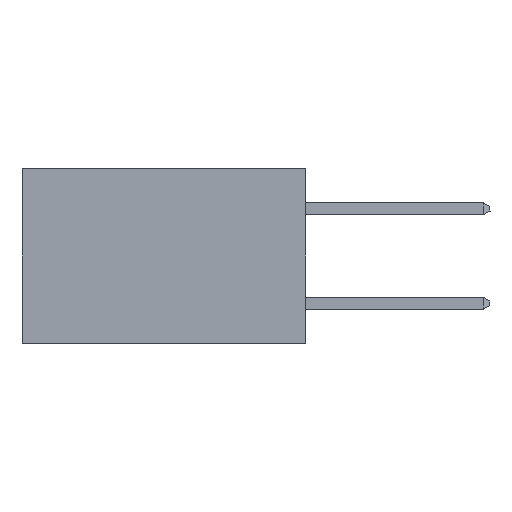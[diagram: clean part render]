
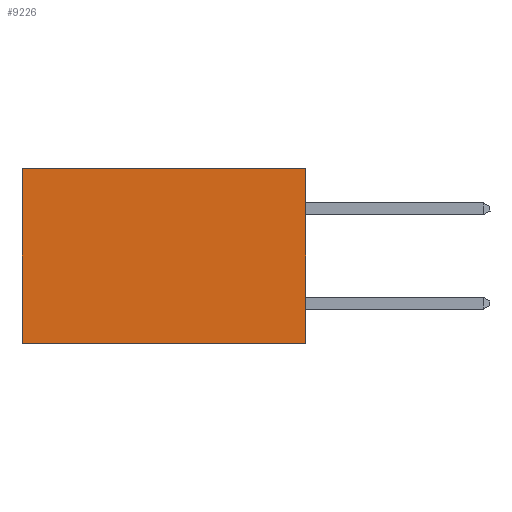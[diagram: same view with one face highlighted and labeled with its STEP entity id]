
A CAD part, left-side view. The second image highlights one B-rep face of the part: STEP entity #9226.
In plain terms, the highlighted planar face has unit normal (-1, 0, 0).
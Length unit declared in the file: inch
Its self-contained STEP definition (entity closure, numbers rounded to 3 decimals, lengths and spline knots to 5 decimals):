
#506 = DIRECTION ( 'NONE',  ( 0., 1., 0. ) ) ;
#550 = EDGE_CURVE ( 'NONE', #14783, #10719, #13028, .T. ) ;
#842 = EDGE_CURVE ( 'NONE', #10719, #13109, #15501, .T. ) ;
#994 = VECTOR ( 'NONE', #506, 39.37008 ) ;
#1002 = EDGE_CURVE ( 'NONE', #3822, #13109, #2439, .T. ) ;
#1236 = FACE_OUTER_BOUND ( 'NONE', #16399, .T. ) ;
#1296 = AXIS2_PLACEMENT_3D ( 'NONE', #7543, #8879, #3554 ) ;
#2439 = LINE ( 'NONE', #15503, #12427 ) ;
#3278 = ORIENTED_EDGE ( 'NONE', *, *, #842, .F. ) ;
#3554 = DIRECTION ( 'NONE',  ( 0., 0., -1. ) ) ;
#3822 = VERTEX_POINT ( 'NONE', #11795 ) ;
#5274 = CARTESIAN_POINT ( 'NONE',  ( 0.298, 0., 0. ) ) ;
#7299 = ORIENTED_EDGE ( 'NONE', *, *, #550, .F. ) ;
#7385 = ORIENTED_EDGE ( 'NONE', *, *, #14530, .T. ) ;
#7543 = CARTESIAN_POINT ( 'NONE',  ( 0.298, 0., 0. ) ) ;
#7677 = DIRECTION ( 'NONE',  ( 0., 0., -1. ) ) ;
#8879 = DIRECTION ( 'NONE',  ( 1., 0., 0. ) ) ;
#8981 = VECTOR ( 'NONE', #12242, 39.37008 ) ;
#9226 = ADVANCED_FACE ( 'NONE', ( #1236 ), #14047, .F. ) ;
#10137 = CARTESIAN_POINT ( 'NONE',  ( 0.298, 0., -0.37 ) ) ;
#10560 = CARTESIAN_POINT ( 'NONE',  ( 0.298, 0., 0. ) ) ;
#10681 = DIRECTION ( 'NONE',  ( 0., 0., -1. ) ) ;
#10719 = VERTEX_POINT ( 'NONE', #13956 ) ;
#10819 = VECTOR ( 'NONE', #10681, 39.37008 ) ;
#11795 = CARTESIAN_POINT ( 'NONE',  ( 0.298, 0.6, 0. ) ) ;
#11883 = CARTESIAN_POINT ( 'NONE',  ( 0.298, 0.6, -0.37 ) ) ;
#12242 = DIRECTION ( 'NONE',  ( 0., 1., 0. ) ) ;
#12427 = VECTOR ( 'NONE', #7677, 39.37008 ) ;
#13028 = LINE ( 'NONE', #10560, #10819 ) ;
#13109 = VERTEX_POINT ( 'NONE', #11883 ) ;
#13585 = LINE ( 'NONE', #15730, #994 ) ;
#13952 = ORIENTED_EDGE ( 'NONE', *, *, #1002, .T. ) ;
#13956 = CARTESIAN_POINT ( 'NONE',  ( 0.298, 0., -0.37 ) ) ;
#14047 = PLANE ( 'NONE',  #1296 ) ;
#14530 = EDGE_CURVE ( 'NONE', #14783, #3822, #13585, .T. ) ;
#14783 = VERTEX_POINT ( 'NONE', #5274 ) ;
#15501 = LINE ( 'NONE', #10137, #8981 ) ;
#15503 = CARTESIAN_POINT ( 'NONE',  ( 0.298, 0.6, 0. ) ) ;
#15730 = CARTESIAN_POINT ( 'NONE',  ( 0.298, 0., 0. ) ) ;
#16399 = EDGE_LOOP ( 'NONE', ( #13952, #3278, #7299, #7385 ) ) ;
